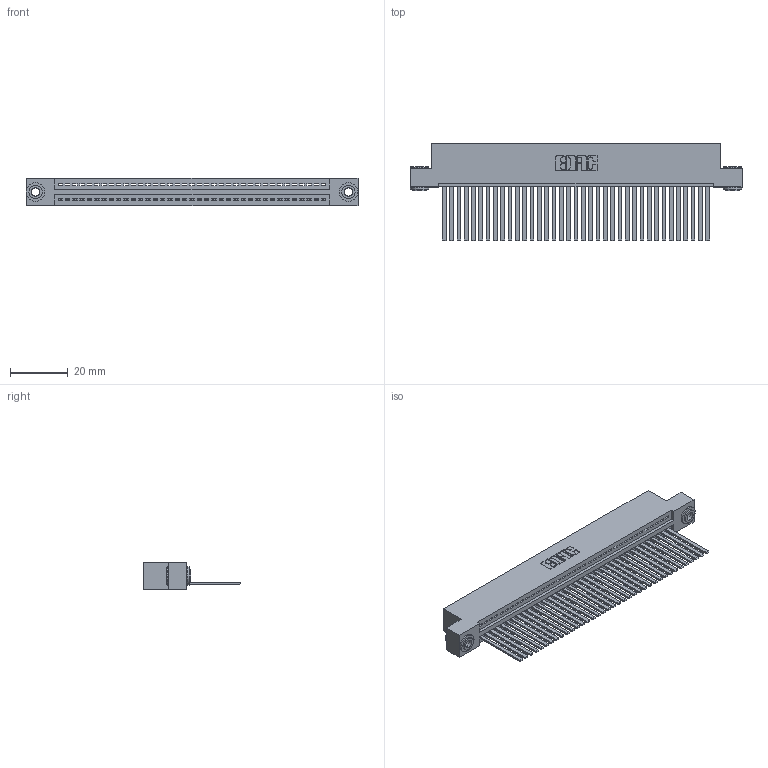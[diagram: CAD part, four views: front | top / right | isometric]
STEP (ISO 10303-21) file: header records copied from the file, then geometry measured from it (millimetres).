
FILE_DESCRIPTION (( 'STEP AP203' ), '1' );
FILE_NAME ('395-037-544-103.STEP', '2018-11-14T00:14:49', ( '' ), ( '' ), 'SwSTEP 2.0', 'SolidWorks 2016', '' );
FILE_SCHEMA (( 'CONFIG_CONTROL_DESIGN' ));
Length unit declared in the file: inch
Products named in the file (4): 345-250-002_345-250-002-102; 345 Part_Flush Mounting Lugs - 0.156 Dia-TH; 395-037-544-103; 345-292-001_345-293-144
Assembly tree (40 placements, depth 2):
  395-037-544-103
    345 Part_Flush Mounting Lugs - 0.156 Dia-TH
    345-292-001_345-293-144  x37
    345-250-002_345-250-002-102  x2
Bounding box: 115.19 x 33.96 x 9.4 mm (x, y, z)
Volume: 11347.7 mm3; surface area: 16513 mm2
Topology: 40 solids, 40 shells, 2088 faces, 6263 edges, 4122 vertices
Faces by surface type: plane 1422, cylinder 658, cone 8
Entity records: 28986 total; most frequent: CARTESIAN_POINT 4998, ORIENTED_EDGE 4962, DIRECTION 4401, EDGE_CURVE 2481, LINE 2181, VECTOR 2181, VERTEX_POINT 1650, AXIS2_PLACEMENT_3D 1110
